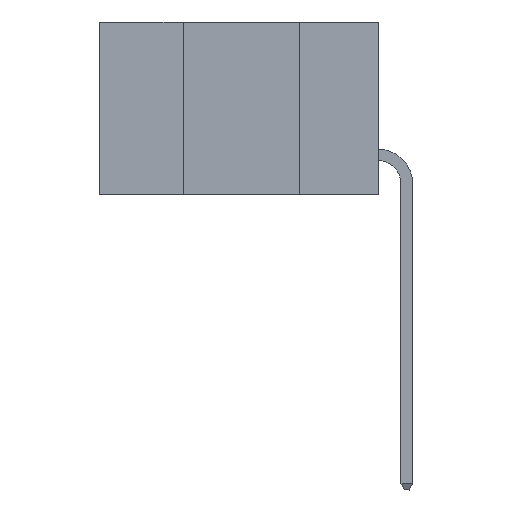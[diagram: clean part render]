
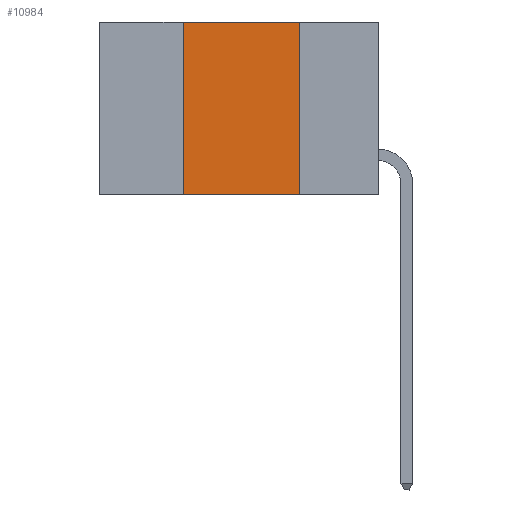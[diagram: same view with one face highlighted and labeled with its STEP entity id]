
A CAD part, left-side view. The second image highlights one B-rep face of the part: STEP entity #10984.
In plain terms, the highlighted planar face has unit normal (-1, 0, 0).
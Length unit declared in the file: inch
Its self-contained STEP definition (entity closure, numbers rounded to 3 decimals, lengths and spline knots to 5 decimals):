
#782 = CARTESIAN_POINT ( 'NONE',  ( 0., 0.42, -0.37 ) ) ;
#1964 = EDGE_CURVE ( 'NONE', #6248, #19756, #15453, .T. ) ;
#2130 = DIRECTION ( 'NONE',  ( 0., 0., -1. ) ) ;
#4376 = PLANE ( 'NONE',  #20013 ) ;
#4436 = ORIENTED_EDGE ( 'NONE', *, *, #1964, .T. ) ;
#4561 = ORIENTED_EDGE ( 'NONE', *, *, #11212, .F. ) ;
#6248 = VERTEX_POINT ( 'NONE', #782 ) ;
#6770 = CARTESIAN_POINT ( 'NONE',  ( 0., 0.17, 0. ) ) ;
#7074 = VECTOR ( 'NONE', #2130, 39.37008 ) ;
#8260 = EDGE_CURVE ( 'NONE', #22184, #21881, #17522, .T. ) ;
#8281 = FACE_OUTER_BOUND ( 'NONE', #15355, .T. ) ;
#8571 = CARTESIAN_POINT ( 'NONE',  ( 0., 0.17, -0.37 ) ) ;
#9610 = CARTESIAN_POINT ( 'NONE',  ( 0., 0.42, -0.37 ) ) ;
#9632 = EDGE_CURVE ( 'NONE', #21881, #19756, #9677, .T. ) ;
#9677 = LINE ( 'NONE', #13860, #7074 ) ;
#10002 = CARTESIAN_POINT ( 'NONE',  ( 0., 0.6, -0.37 ) ) ;
#10017 = VECTOR ( 'NONE', #11699, 39.37008 ) ;
#10984 = ADVANCED_FACE ( 'NONE', ( #8281 ), #4376, .F. ) ;
#11212 = EDGE_CURVE ( 'NONE', #6248, #22184, #13677, .T. ) ;
#11699 = DIRECTION ( 'NONE',  ( 0., -1., 0. ) ) ;
#12081 = DIRECTION ( 'NONE',  ( 1., 0., 0. ) ) ;
#13677 = LINE ( 'NONE', #9610, #14407 ) ;
#13860 = CARTESIAN_POINT ( 'NONE',  ( 0., 0.17, -0.37 ) ) ;
#14228 = CARTESIAN_POINT ( 'NONE',  ( 0., 0.6, 0. ) ) ;
#14407 = VECTOR ( 'NONE', #17827, 39.37008 ) ;
#15355 = EDGE_LOOP ( 'NONE', ( #16754, #20091, #4561, #4436 ) ) ;
#15453 = LINE ( 'NONE', #10002, #23190 ) ;
#16754 = ORIENTED_EDGE ( 'NONE', *, *, #9632, .F. ) ;
#17027 = CARTESIAN_POINT ( 'NONE',  ( 0., 0.6, 0. ) ) ;
#17522 = LINE ( 'NONE', #17027, #10017 ) ;
#17723 = DIRECTION ( 'NONE',  ( 0., -1., 0. ) ) ;
#17827 = DIRECTION ( 'NONE',  ( 0., 0., 1. ) ) ;
#19756 = VERTEX_POINT ( 'NONE', #8571 ) ;
#19779 = DIRECTION ( 'NONE',  ( 0., 0., -1. ) ) ;
#20013 = AXIS2_PLACEMENT_3D ( 'NONE', #14228, #12081, #19779 ) ;
#20091 = ORIENTED_EDGE ( 'NONE', *, *, #8260, .F. ) ;
#21245 = CARTESIAN_POINT ( 'NONE',  ( 0., 0.42, 0. ) ) ;
#21881 = VERTEX_POINT ( 'NONE', #6770 ) ;
#22184 = VERTEX_POINT ( 'NONE', #21245 ) ;
#23190 = VECTOR ( 'NONE', #17723, 39.37008 ) ;
